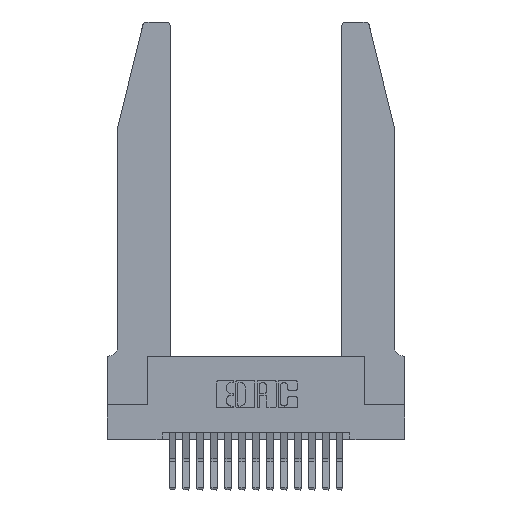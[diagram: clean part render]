
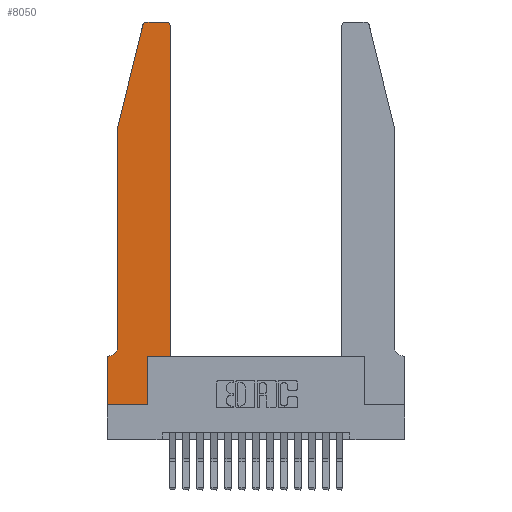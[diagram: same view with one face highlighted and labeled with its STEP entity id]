
A CAD part, top view. The second image highlights one B-rep face of the part: STEP entity #8050.
In plain terms, the highlighted planar face has unit normal (0, 0, 1).
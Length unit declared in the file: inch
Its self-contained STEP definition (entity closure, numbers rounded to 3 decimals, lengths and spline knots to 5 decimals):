
#328 = DIRECTION ( 'NONE',  ( -0.239, -0.971, 0. ) ) ;
#1227 = VERTEX_POINT ( 'NONE', #17175 ) ;
#1586 = EDGE_CURVE ( 'NONE', #6870, #7615, #3659, .T. ) ;
#1617 = DIRECTION ( 'NONE',  ( 0., 0., 1. ) ) ;
#1677 = DIRECTION ( 'NONE',  ( 1., 0., 0. ) ) ;
#1849 = VECTOR ( 'NONE', #3751, 39.37008 ) ;
#2216 = AXIS2_PLACEMENT_3D ( 'NONE', #5299, #6894, #18555 ) ;
#2227 = CARTESIAN_POINT ( 'NONE',  ( 0.2865, 0., 0.37 ) ) ;
#2276 = ORIENTED_EDGE ( 'NONE', *, *, #6103, .T. ) ;
#2429 = CARTESIAN_POINT ( 'NONE',  ( 0.2605, 2.75, 0.37 ) ) ;
#2618 = ORIENTED_EDGE ( 'NONE', *, *, #3242, .T. ) ;
#2635 = ORIENTED_EDGE ( 'NONE', *, *, #9583, .T. ) ;
#2736 = LINE ( 'NONE', #7484, #13041 ) ;
#2810 = CARTESIAN_POINT ( 'NONE',  ( 0.0055, 0.42, 0.37 ) ) ;
#3014 = CARTESIAN_POINT ( 'NONE',  ( 0.4205, 2.72, 0.37 ) ) ;
#3242 = EDGE_CURVE ( 'NONE', #1227, #6870, #2736, .T. ) ;
#3510 = CARTESIAN_POINT ( 'NONE',  ( 0.284, 2.75, 0.37 ) ) ;
#3659 = LINE ( 'NONE', #4911, #1849 ) ;
#3751 = DIRECTION ( 'NONE',  ( 0., -1., 0. ) ) ;
#3792 = DIRECTION ( 'NONE',  ( 0., -1., 0. ) ) ;
#4381 = LINE ( 'NONE', #18117, #14914 ) ;
#4559 = CARTESIAN_POINT ( 'NONE',  ( 0.0755, 2., 0.37 ) ) ;
#4672 = LINE ( 'NONE', #7890, #6722 ) ;
#4911 = CARTESIAN_POINT ( 'NONE',  ( 0., 0., 0.37 ) ) ;
#5105 = DIRECTION ( 'NONE',  ( 1., 0., 0. ) ) ;
#5220 = AXIS2_PLACEMENT_3D ( 'NONE', #6178, #17884, #10536 ) ;
#5299 = CARTESIAN_POINT ( 'NONE',  ( 0., 0.35, 0.37 ) ) ;
#5356 = ORIENTED_EDGE ( 'NONE', *, *, #1586, .T. ) ;
#6103 = EDGE_CURVE ( 'NONE', #17728, #1227, #11326, .T. ) ;
#6125 = ORIENTED_EDGE ( 'NONE', *, *, #8772, .T. ) ;
#6178 = CARTESIAN_POINT ( 'NONE',  ( 0.284, 2.72, 0.37 ) ) ;
#6722 = VECTOR ( 'NONE', #16748, 39.37008 ) ;
#6870 = VERTEX_POINT ( 'NONE', #9301 ) ;
#6894 = DIRECTION ( 'NONE',  ( 0., 0., 1. ) ) ;
#7148 = LINE ( 'NONE', #16929, #11931 ) ;
#7292 = EDGE_CURVE ( 'NONE', #9740, #11183, #4672, .T. ) ;
#7392 = FACE_OUTER_BOUND ( 'NONE', #15929, .T. ) ;
#7475 = CARTESIAN_POINT ( 'NONE',  ( 0., 0., 0.37 ) ) ;
#7484 = CARTESIAN_POINT ( 'NONE',  ( 0.0755, 0.35, 0.37 ) ) ;
#7579 = DIRECTION ( 'NONE',  ( 0., 1., 0. ) ) ;
#7615 = VERTEX_POINT ( 'NONE', #7475 ) ;
#7890 = CARTESIAN_POINT ( 'NONE',  ( 0.4505, 0.35, 0.37 ) ) ;
#7942 = ORIENTED_EDGE ( 'NONE', *, *, #13291, .T. ) ;
#8011 = LINE ( 'NONE', #13803, #8923 ) ;
#8050 = ADVANCED_FACE ( 'NONE', ( #7392 ), #17080, .T. ) ;
#8239 = CARTESIAN_POINT ( 'NONE',  ( 0.4505, 0.35, 0.37 ) ) ;
#8394 = VERTEX_POINT ( 'NONE', #16693 ) ;
#8772 = EDGE_CURVE ( 'NONE', #14758, #17728, #7148, .T. ) ;
#8923 = VECTOR ( 'NONE', #5105, 39.37008 ) ;
#9169 = CIRCLE ( 'NONE', #5220, 0.03 ) ;
#9229 = ORIENTED_EDGE ( 'NONE', *, *, #7292, .T. ) ;
#9301 = CARTESIAN_POINT ( 'NONE',  ( 0., 0.35, 0.37 ) ) ;
#9305 = VERTEX_POINT ( 'NONE', #3510 ) ;
#9502 = CARTESIAN_POINT ( 'NONE',  ( 0.2865, 0.35, 0.37 ) ) ;
#9583 = EDGE_CURVE ( 'NONE', #7615, #17545, #8011, .T. ) ;
#9736 = EDGE_CURVE ( 'NONE', #16117, #9305, #10972, .T. ) ;
#9740 = VERTEX_POINT ( 'NONE', #9502 ) ;
#9879 = DIRECTION ( 'NONE',  ( -1., 0., 0. ) ) ;
#10536 = DIRECTION ( 'NONE',  ( 1., 0., 0. ) ) ;
#10625 = AXIS2_PLACEMENT_3D ( 'NONE', #2810, #18701, #9879 ) ;
#10697 = AXIS2_PLACEMENT_3D ( 'NONE', #3014, #1617, #1677 ) ;
#10972 = LINE ( 'NONE', #2429, #14678 ) ;
#11183 = VERTEX_POINT ( 'NONE', #8239 ) ;
#11326 = CIRCLE ( 'NONE', #10625, 0.07 ) ;
#11931 = VECTOR ( 'NONE', #3792, 39.37008 ) ;
#12109 = ORIENTED_EDGE ( 'NONE', *, *, #18282, .T. ) ;
#12606 = LINE ( 'NONE', #13105, #17644 ) ;
#13041 = VECTOR ( 'NONE', #17749, 39.37008 ) ;
#13047 = EDGE_CURVE ( 'NONE', #9305, #8394, #9169, .T. ) ;
#13105 = CARTESIAN_POINT ( 'NONE',  ( 0.2865, 0.35, 0.37 ) ) ;
#13291 = EDGE_CURVE ( 'NONE', #18340, #16117, #17450, .T. ) ;
#13546 = EDGE_CURVE ( 'NONE', #8394, #14758, #4381, .T. ) ;
#13803 = CARTESIAN_POINT ( 'NONE',  ( 0., 0., 0.37 ) ) ;
#13858 = CARTESIAN_POINT ( 'NONE',  ( 0.4205, 2.75, 0.37 ) ) ;
#14095 = EDGE_CURVE ( 'NONE', #11183, #18340, #14174, .T. ) ;
#14174 = LINE ( 'NONE', #14904, #18552 ) ;
#14678 = VECTOR ( 'NONE', #18510, 39.37008 ) ;
#14758 = VERTEX_POINT ( 'NONE', #4559 ) ;
#14904 = CARTESIAN_POINT ( 'NONE',  ( 0.4505, 0.35, 0.37 ) ) ;
#14914 = VECTOR ( 'NONE', #328, 39.37008 ) ;
#15903 = ORIENTED_EDGE ( 'NONE', *, *, #14095, .T. ) ;
#15929 = EDGE_LOOP ( 'NONE', ( #16844, #17614, #16879, #6125, #2276, #2618, #5356, #2635, #12109, #9229, #15903, #7942 ) ) ;
#16117 = VERTEX_POINT ( 'NONE', #13858 ) ;
#16693 = CARTESIAN_POINT ( 'NONE',  ( 0.25487, 2.72718, 0.37 ) ) ;
#16748 = DIRECTION ( 'NONE',  ( 1., 0., 0. ) ) ;
#16844 = ORIENTED_EDGE ( 'NONE', *, *, #9736, .T. ) ;
#16879 = ORIENTED_EDGE ( 'NONE', *, *, #13546, .T. ) ;
#16929 = CARTESIAN_POINT ( 'NONE',  ( 0.0755, 2., 0.37 ) ) ;
#17080 = PLANE ( 'NONE',  #2216 ) ;
#17175 = CARTESIAN_POINT ( 'NONE',  ( 0.0055, 0.35, 0.37 ) ) ;
#17203 = DIRECTION ( 'NONE',  ( 0., 1., 0. ) ) ;
#17450 = CIRCLE ( 'NONE', #10697, 0.03 ) ;
#17545 = VERTEX_POINT ( 'NONE', #2227 ) ;
#17614 = ORIENTED_EDGE ( 'NONE', *, *, #13047, .T. ) ;
#17644 = VECTOR ( 'NONE', #17203, 39.37008 ) ;
#17711 = CARTESIAN_POINT ( 'NONE',  ( 0.4505, 2.72, 0.37 ) ) ;
#17728 = VERTEX_POINT ( 'NONE', #18952 ) ;
#17749 = DIRECTION ( 'NONE',  ( -1., 0., 0. ) ) ;
#17884 = DIRECTION ( 'NONE',  ( 0., 0., 1. ) ) ;
#18117 = CARTESIAN_POINT ( 'NONE',  ( 0.0755, 2., 0.37 ) ) ;
#18282 = EDGE_CURVE ( 'NONE', #17545, #9740, #12606, .T. ) ;
#18340 = VERTEX_POINT ( 'NONE', #17711 ) ;
#18510 = DIRECTION ( 'NONE',  ( -1., 0., 0. ) ) ;
#18552 = VECTOR ( 'NONE', #7579, 39.37008 ) ;
#18555 = DIRECTION ( 'NONE',  ( 1., 0., 0. ) ) ;
#18701 = DIRECTION ( 'NONE',  ( 0., 0., -1. ) ) ;
#18952 = CARTESIAN_POINT ( 'NONE',  ( 0.0755, 0.42, 0.37 ) ) ;
